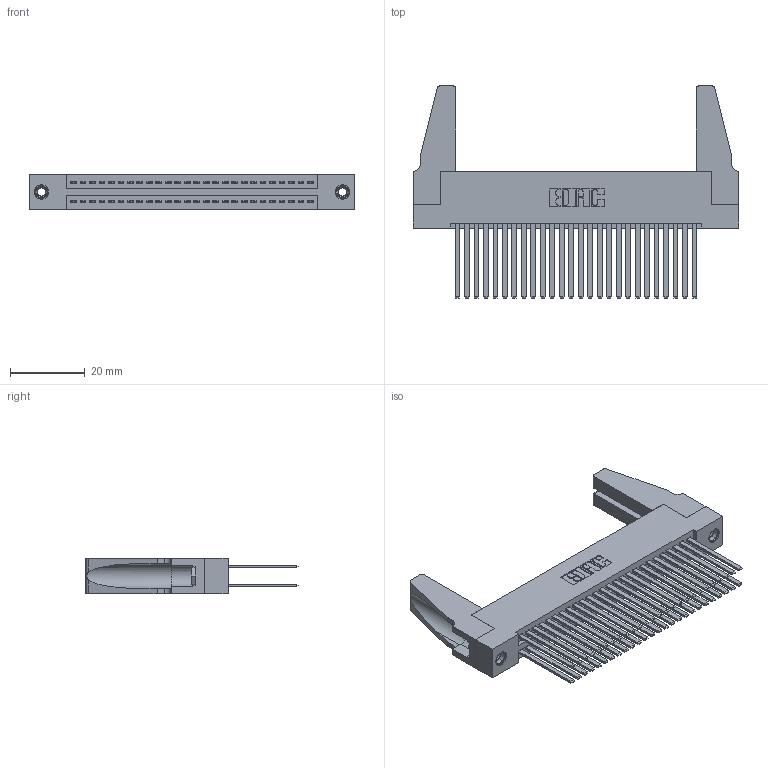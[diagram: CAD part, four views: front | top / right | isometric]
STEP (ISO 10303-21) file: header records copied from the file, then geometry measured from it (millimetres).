
FILE_DESCRIPTION (( 'STEP AP203' ), '1' );
FILE_NAME ('345-052-544-288.STEP', '2019-10-29T16:57:28', ( '' ), ( '' ), 'SwSTEP 2.0', 'SolidWorks 2016', '' );
FILE_SCHEMA (( 'CONFIG_CONTROL_DESIGN' ));
Length unit declared in the file: inch
Products named in the file (5): 345-250-001_345-250-001-102; 345-292-001_345-293-144; 345-052-544-288; 345-220-078_345-220-088; 345 Part_Flush Mounting Lugs - 0.156 Dia-TH
Assembly tree (57 placements, depth 2):
  345-052-544-288
    345 Part_Flush Mounting Lugs - 0.156 Dia-TH
    345-292-001_345-293-144  x52
    345-250-001_345-250-001-102  x2
    345-220-078_345-220-088  x2
Bounding box: 87.27 x 56.82 x 9.4 mm (x, y, z)
Volume: 12310.8 mm3; surface area: 18338.5 mm2
Topology: 57 solids, 57 shells, 2538 faces, 7467 edges, 4898 vertices
Faces by surface type: plane 1660, cylinder 862, cone 12, torus 4
Entity records: 24518 total; most frequent: CARTESIAN_POINT 4118, ORIENTED_EDGE 4012, DIRECTION 3654, EDGE_CURVE 2006, VECTOR 1732, LINE 1732, VERTEX_POINT 1330, AXIS2_PLACEMENT_3D 961
